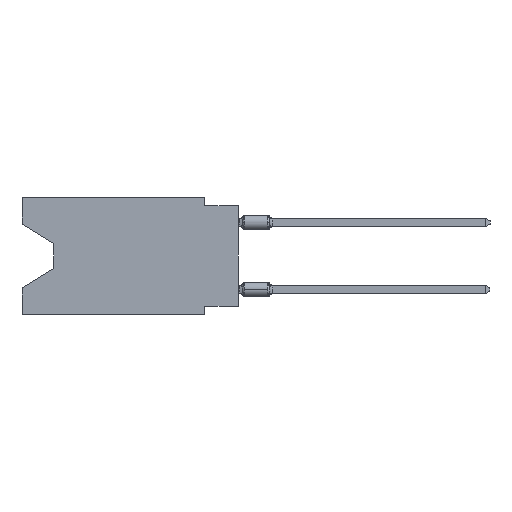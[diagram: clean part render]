
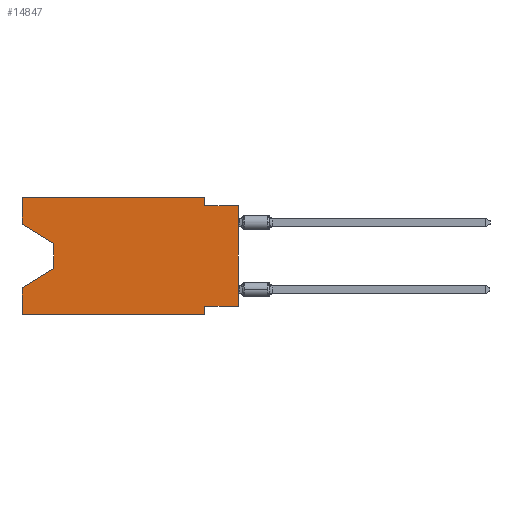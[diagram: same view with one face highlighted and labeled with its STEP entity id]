
A CAD part, left-side view. The second image highlights one B-rep face of the part: STEP entity #14847.
In plain terms, the highlighted planar face has unit normal (-1, 0, 0).
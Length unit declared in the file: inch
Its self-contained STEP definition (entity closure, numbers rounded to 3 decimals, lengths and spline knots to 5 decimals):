
#65 = EDGE_CURVE ( 'NONE', #9338, #9300, #9969, .T. ) ;
#125 = LINE ( 'NONE', #9267, #10127 ) ;
#212 = CARTESIAN_POINT ( 'NONE',  ( 0., 0.645, -0.08025 ) ) ;
#226 = VECTOR ( 'NONE', #5241, 39.37008 ) ;
#238 = CARTESIAN_POINT ( 'NONE',  ( 0., 0., -0.325 ) ) ;
#254 = VERTEX_POINT ( 'NONE', #6019 ) ;
#919 = PLANE ( 'NONE',  #4583 ) ;
#1531 = EDGE_CURVE ( 'NONE', #1721, #10382, #2782, .T. ) ;
#1721 = VERTEX_POINT ( 'NONE', #3471 ) ;
#1921 = VERTEX_POINT ( 'NONE', #14411 ) ;
#2442 = EDGE_LOOP ( 'NONE', ( #4999, #11110, #12744, #6605, #2588, #10265, #4339, #11941, #8281, #12288, #12794, #13397 ) ) ;
#2575 = DIRECTION ( 'NONE',  ( 0., -1., 0. ) ) ;
#2588 = ORIENTED_EDGE ( 'NONE', *, *, #1531, .T. ) ;
#2730 = EDGE_CURVE ( 'NONE', #12563, #9338, #12257, .T. ) ;
#2782 = LINE ( 'NONE', #9931, #12190 ) ;
#2787 = LINE ( 'NONE', #7464, #10141 ) ;
#3119 = VERTEX_POINT ( 'NONE', #238 ) ;
#3471 = CARTESIAN_POINT ( 'NONE',  ( 0., 0.645, -0.35 ) ) ;
#3708 = CARTESIAN_POINT ( 'NONE',  ( 0., 0.1, -0.35 ) ) ;
#3880 = CARTESIAN_POINT ( 'NONE',  ( 0., 0.645, 0. ) ) ;
#3917 = VERTEX_POINT ( 'NONE', #13755 ) ;
#3980 = LINE ( 'NONE', #14556, #11275 ) ;
#3986 = VECTOR ( 'NONE', #14704, 39.37008 ) ;
#4115 = CARTESIAN_POINT ( 'NONE',  ( 0., 0., -0.025 ) ) ;
#4210 = DIRECTION ( 'NONE',  ( 1., 0., 0. ) ) ;
#4339 = ORIENTED_EDGE ( 'NONE', *, *, #11042, .F. ) ;
#4459 = CARTESIAN_POINT ( 'NONE',  ( 0., 0.645, 0. ) ) ;
#4583 = AXIS2_PLACEMENT_3D ( 'NONE', #7981, #4210, #13633 ) ;
#4812 = LINE ( 'NONE', #9431, #8819 ) ;
#4843 = CARTESIAN_POINT ( 'NONE',  ( 0., 0.1, 0. ) ) ;
#4934 = LINE ( 'NONE', #14122, #11847 ) ;
#4985 = VECTOR ( 'NONE', #2575, 39.37008 ) ;
#4999 = ORIENTED_EDGE ( 'NONE', *, *, #9051, .T. ) ;
#5010 = CARTESIAN_POINT ( 'NONE',  ( 0., 0.645, 0. ) ) ;
#5241 = DIRECTION ( 'NONE',  ( 0., 0., -1. ) ) ;
#5376 = DIRECTION ( 'NONE',  ( 0., 0., 1. ) ) ;
#5509 = FACE_OUTER_BOUND ( 'NONE', #2442, .T. ) ;
#6019 = CARTESIAN_POINT ( 'NONE',  ( 0., 0.645, -0.26975 ) ) ;
#6150 = LINE ( 'NONE', #3708, #11379 ) ;
#6475 = VECTOR ( 'NONE', #5376, 39.37008 ) ;
#6605 = ORIENTED_EDGE ( 'NONE', *, *, #13255, .F. ) ;
#6614 = DIRECTION ( 'NONE',  ( 0., 0., 1. ) ) ;
#7394 = EDGE_CURVE ( 'NONE', #10254, #12917, #8202, .T. ) ;
#7464 = CARTESIAN_POINT ( 'NONE',  ( 0., 0., 0. ) ) ;
#7526 = EDGE_CURVE ( 'NONE', #1921, #254, #3980, .T. ) ;
#7981 = CARTESIAN_POINT ( 'NONE',  ( 0., 0.645, 0. ) ) ;
#8202 = LINE ( 'NONE', #13158, #10283 ) ;
#8281 = ORIENTED_EDGE ( 'NONE', *, *, #65, .F. ) ;
#8727 = DIRECTION ( 'NONE',  ( 0., 0.855, -0.519 ) ) ;
#8792 = CARTESIAN_POINT ( 'NONE',  ( 0., 0.1, -0.025 ) ) ;
#8819 = VECTOR ( 'NONE', #10508, 39.37008 ) ;
#8957 = CARTESIAN_POINT ( 'NONE',  ( 0., 0., -0.025 ) ) ;
#9051 = EDGE_CURVE ( 'NONE', #10254, #10704, #4812, .T. ) ;
#9267 = CARTESIAN_POINT ( 'NONE',  ( 0., 0.55, -0.138 ) ) ;
#9300 = VERTEX_POINT ( 'NONE', #4115 ) ;
#9338 = VERTEX_POINT ( 'NONE', #8792 ) ;
#9431 = CARTESIAN_POINT ( 'NONE',  ( 0., 0.645, -0.08025 ) ) ;
#9931 = CARTESIAN_POINT ( 'NONE',  ( 0., 0.645, -0.35 ) ) ;
#9935 = CARTESIAN_POINT ( 'NONE',  ( 0., 0.1, 0. ) ) ;
#9969 = LINE ( 'NONE', #8957, #3986 ) ;
#10127 = VECTOR ( 'NONE', #12691, 39.37008 ) ;
#10141 = VECTOR ( 'NONE', #6614, 39.37008 ) ;
#10254 = VERTEX_POINT ( 'NONE', #212 ) ;
#10265 = ORIENTED_EDGE ( 'NONE', *, *, #14239, .F. ) ;
#10283 = VECTOR ( 'NONE', #11845, 39.37008 ) ;
#10382 = VERTEX_POINT ( 'NONE', #14778 ) ;
#10384 = LINE ( 'NONE', #4459, #6475 ) ;
#10508 = DIRECTION ( 'NONE',  ( 0., -0.855, -0.519 ) ) ;
#10704 = VERTEX_POINT ( 'NONE', #12122 ) ;
#10855 = DIRECTION ( 'NONE',  ( 0., 0., -1. ) ) ;
#11042 = EDGE_CURVE ( 'NONE', #3119, #3917, #4934, .T. ) ;
#11110 = ORIENTED_EDGE ( 'NONE', *, *, #11613, .T. ) ;
#11275 = VECTOR ( 'NONE', #8727, 39.37008 ) ;
#11379 = VECTOR ( 'NONE', #10855, 39.37008 ) ;
#11613 = EDGE_CURVE ( 'NONE', #10704, #1921, #125, .T. ) ;
#11845 = DIRECTION ( 'NONE',  ( 0., 0., 1. ) ) ;
#11847 = VECTOR ( 'NONE', #13267, 39.37008 ) ;
#11941 = ORIENTED_EDGE ( 'NONE', *, *, #12324, .T. ) ;
#12122 = CARTESIAN_POINT ( 'NONE',  ( 0., 0.55, -0.138 ) ) ;
#12190 = VECTOR ( 'NONE', #14663, 39.37008 ) ;
#12257 = LINE ( 'NONE', #9935, #226 ) ;
#12288 = ORIENTED_EDGE ( 'NONE', *, *, #2730, .F. ) ;
#12324 = EDGE_CURVE ( 'NONE', #3119, #9300, #2787, .T. ) ;
#12563 = VERTEX_POINT ( 'NONE', #4843 ) ;
#12691 = DIRECTION ( 'NONE',  ( 0., 0., -1. ) ) ;
#12744 = ORIENTED_EDGE ( 'NONE', *, *, #7526, .T. ) ;
#12794 = ORIENTED_EDGE ( 'NONE', *, *, #13685, .F. ) ;
#12917 = VERTEX_POINT ( 'NONE', #5010 ) ;
#13133 = LINE ( 'NONE', #3880, #4985 ) ;
#13158 = CARTESIAN_POINT ( 'NONE',  ( 0., 0.645, 0. ) ) ;
#13255 = EDGE_CURVE ( 'NONE', #1721, #254, #10384, .T. ) ;
#13267 = DIRECTION ( 'NONE',  ( 0., 1., 0. ) ) ;
#13397 = ORIENTED_EDGE ( 'NONE', *, *, #7394, .F. ) ;
#13633 = DIRECTION ( 'NONE',  ( 0., 0., -1. ) ) ;
#13685 = EDGE_CURVE ( 'NONE', #12917, #12563, #13133, .T. ) ;
#13755 = CARTESIAN_POINT ( 'NONE',  ( 0., 0.1, -0.325 ) ) ;
#14122 = CARTESIAN_POINT ( 'NONE',  ( 0., 0., -0.325 ) ) ;
#14239 = EDGE_CURVE ( 'NONE', #3917, #10382, #6150, .T. ) ;
#14411 = CARTESIAN_POINT ( 'NONE',  ( 0., 0.55, -0.212 ) ) ;
#14556 = CARTESIAN_POINT ( 'NONE',  ( 0., 0.55, -0.212 ) ) ;
#14663 = DIRECTION ( 'NONE',  ( 0., -1., 0. ) ) ;
#14704 = DIRECTION ( 'NONE',  ( 0., -1., 0. ) ) ;
#14778 = CARTESIAN_POINT ( 'NONE',  ( 0., 0.1, -0.35 ) ) ;
#14847 = ADVANCED_FACE ( 'NONE', ( #5509 ), #919, .F. ) ;
